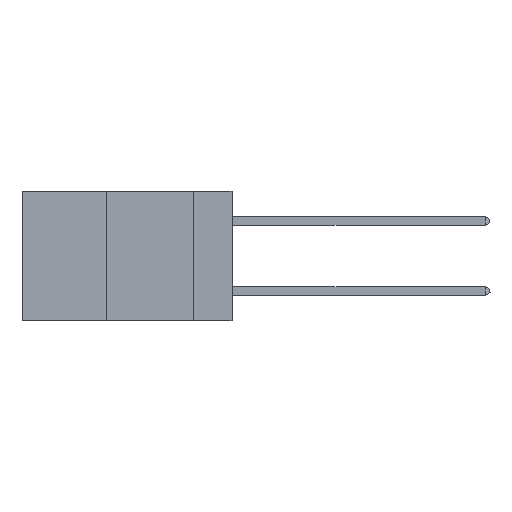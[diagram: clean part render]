
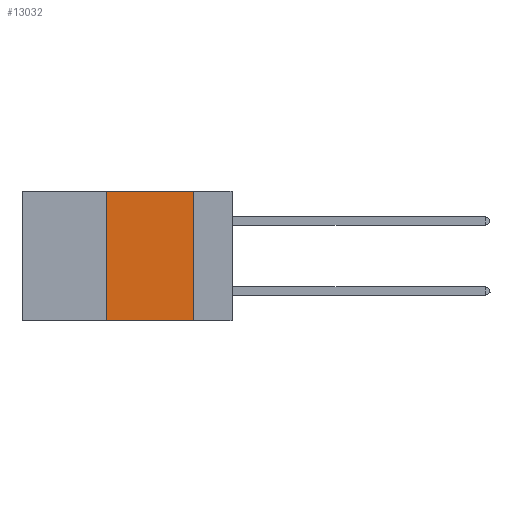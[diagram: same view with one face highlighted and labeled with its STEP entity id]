
A CAD part, left-side view. The second image highlights one B-rep face of the part: STEP entity #13032.
In plain terms, the highlighted planar face has unit normal (-1, 0, 0).
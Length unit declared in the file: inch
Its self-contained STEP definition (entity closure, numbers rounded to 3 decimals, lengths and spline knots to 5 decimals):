
#1194 = DIRECTION ( 'NONE',  ( 0., -1., 0. ) ) ;
#1855 = LINE ( 'NONE', #12075, #5904 ) ;
#2032 = DIRECTION ( 'NONE',  ( 1., 0., 0. ) ) ;
#3372 = ORIENTED_EDGE ( 'NONE', *, *, #16501, .F. ) ;
#4206 = AXIS2_PLACEMENT_3D ( 'NONE', #26547, #2032, #23372 ) ;
#5904 = VECTOR ( 'NONE', #9737, 39.37008 ) ;
#6046 = ORIENTED_EDGE ( 'NONE', *, *, #8476, .F. ) ;
#7971 = VECTOR ( 'NONE', #14622, 39.37008 ) ;
#8476 = EDGE_CURVE ( 'NONE', #33645, #26092, #25712, .T. ) ;
#9325 = EDGE_CURVE ( 'NONE', #11413, #24063, #14703, .T. ) ;
#9737 = DIRECTION ( 'NONE',  ( 0., 0., 1. ) ) ;
#11413 = VERTEX_POINT ( 'NONE', #26990 ) ;
#12075 = CARTESIAN_POINT ( 'NONE',  ( 0., 0.36, 0. ) ) ;
#12414 = PLANE ( 'NONE',  #4206 ) ;
#13032 = ADVANCED_FACE ( 'NONE', ( #29217 ), #12414, .F. ) ;
#13949 = VECTOR ( 'NONE', #1194, 39.37008 ) ;
#14622 = DIRECTION ( 'NONE',  ( 0., 0., -1. ) ) ;
#14703 = LINE ( 'NONE', #20111, #27916 ) ;
#15618 = ORIENTED_EDGE ( 'NONE', *, *, #9325, .T. ) ;
#16501 = EDGE_CURVE ( 'NONE', #26092, #24063, #17146, .T. ) ;
#17146 = LINE ( 'NONE', #19680, #7971 ) ;
#19680 = CARTESIAN_POINT ( 'NONE',  ( 0., 0.11, 0. ) ) ;
#19829 = EDGE_CURVE ( 'NONE', #11413, #33645, #1855, .T. ) ;
#20111 = CARTESIAN_POINT ( 'NONE',  ( 0., 0.6, -0.37 ) ) ;
#22024 = CARTESIAN_POINT ( 'NONE',  ( 0., 0.11, -0.37 ) ) ;
#22025 = EDGE_LOOP ( 'NONE', ( #3372, #6046, #26905, #15618 ) ) ;
#23372 = DIRECTION ( 'NONE',  ( 0., 0., -1. ) ) ;
#24063 = VERTEX_POINT ( 'NONE', #22024 ) ;
#25369 = CARTESIAN_POINT ( 'NONE',  ( 0., 0.6, 0. ) ) ;
#25712 = LINE ( 'NONE', #25369, #13949 ) ;
#26092 = VERTEX_POINT ( 'NONE', #29378 ) ;
#26547 = CARTESIAN_POINT ( 'NONE',  ( 0., 0.6, 0. ) ) ;
#26905 = ORIENTED_EDGE ( 'NONE', *, *, #19829, .F. ) ;
#26990 = CARTESIAN_POINT ( 'NONE',  ( 0., 0.36, -0.37 ) ) ;
#27916 = VECTOR ( 'NONE', #30967, 39.37008 ) ;
#29217 = FACE_OUTER_BOUND ( 'NONE', #22025, .T. ) ;
#29378 = CARTESIAN_POINT ( 'NONE',  ( 0., 0.11, 0. ) ) ;
#30967 = DIRECTION ( 'NONE',  ( 0., -1., 0. ) ) ;
#33645 = VERTEX_POINT ( 'NONE', #33715 ) ;
#33715 = CARTESIAN_POINT ( 'NONE',  ( 0., 0.36, 0. ) ) ;
